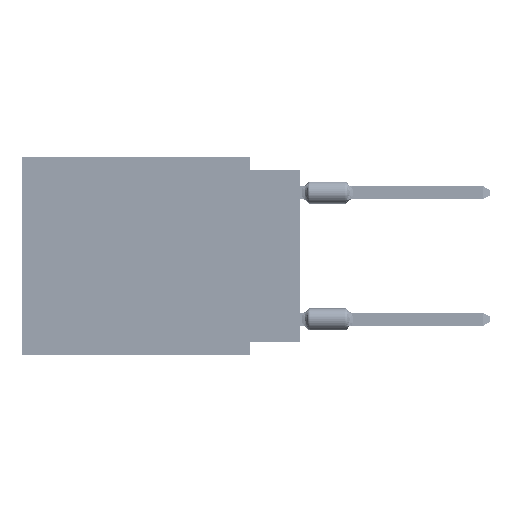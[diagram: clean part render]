
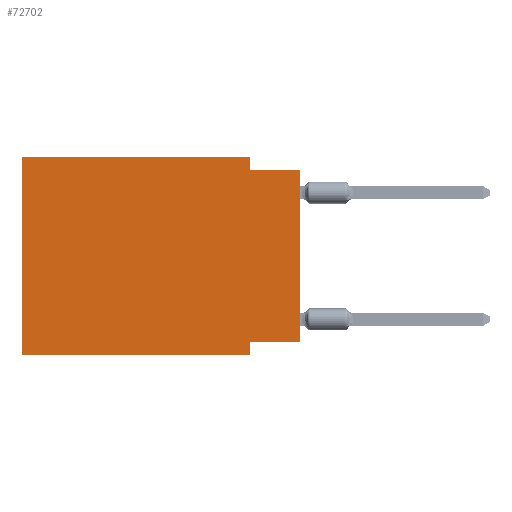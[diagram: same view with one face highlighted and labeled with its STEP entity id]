
A CAD part, left-side view. The second image highlights one B-rep face of the part: STEP entity #72702.
In plain terms, the highlighted planar face has unit normal (-1, 0, 0).
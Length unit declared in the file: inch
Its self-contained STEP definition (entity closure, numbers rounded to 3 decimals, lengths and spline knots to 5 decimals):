
#248 = ORIENTED_EDGE ( 'NONE', *, *, #46616, .F. ) ;
#855 = VERTEX_POINT ( 'NONE', #17338 ) ;
#4907 = EDGE_CURVE ( 'NONE', #21713, #52062, #63877, .T. ) ;
#8021 = VECTOR ( 'NONE', #56955, 39.37008 ) ;
#8079 = VECTOR ( 'NONE', #19343, 39.37008 ) ;
#8705 = DIRECTION ( 'NONE',  ( 0., 0., -1. ) ) ;
#11997 = VERTEX_POINT ( 'NONE', #60979 ) ;
#12090 = VECTOR ( 'NONE', #21885, 39.37008 ) ;
#13390 = ORIENTED_EDGE ( 'NONE', *, *, #50834, .F. ) ;
#13550 = VERTEX_POINT ( 'NONE', #25296 ) ;
#13817 = ORIENTED_EDGE ( 'NONE', *, *, #52555, .T. ) ;
#13846 = CARTESIAN_POINT ( 'NONE',  ( 0., 0., -0.365 ) ) ;
#15242 = AXIS2_PLACEMENT_3D ( 'NONE', #73404, #66898, #30303 ) ;
#16432 = VERTEX_POINT ( 'NONE', #57697 ) ;
#17338 = CARTESIAN_POINT ( 'NONE',  ( 0., 0.1, -0.025 ) ) ;
#18541 = FACE_OUTER_BOUND ( 'NONE', #53073, .T. ) ;
#19343 = DIRECTION ( 'NONE',  ( 0., 0., -1. ) ) ;
#20494 = EDGE_CURVE ( 'NONE', #21713, #43402, #51927, .T. ) ;
#21713 = VERTEX_POINT ( 'NONE', #13846 ) ;
#21885 = DIRECTION ( 'NONE',  ( 0., -1., 0. ) ) ;
#22284 = LINE ( 'NONE', #28752, #12090 ) ;
#22707 = VECTOR ( 'NONE', #46267, 39.37008 ) ;
#23583 = EDGE_CURVE ( 'NONE', #16432, #855, #25038, .T. ) ;
#25038 = LINE ( 'NONE', #44922, #8079 ) ;
#25296 = CARTESIAN_POINT ( 'NONE',  ( 0., 0.55, 0. ) ) ;
#26892 = DIRECTION ( 'NONE',  ( 0., 1., 0. ) ) ;
#27740 = ORIENTED_EDGE ( 'NONE', *, *, #44227, .F. ) ;
#28752 = CARTESIAN_POINT ( 'NONE',  ( 0., 0.55, -0.39 ) ) ;
#28840 = CARTESIAN_POINT ( 'NONE',  ( 0., 0.1, -0.365 ) ) ;
#30303 = DIRECTION ( 'NONE',  ( 0., 0., -1. ) ) ;
#33989 = EDGE_CURVE ( 'NONE', #855, #43402, #34482, .T. ) ;
#34482 = LINE ( 'NONE', #71459, #22707 ) ;
#39446 = LINE ( 'NONE', #63038, #8021 ) ;
#39903 = CARTESIAN_POINT ( 'NONE',  ( 0., 0., -0.365 ) ) ;
#43402 = VERTEX_POINT ( 'NONE', #49380 ) ;
#44103 = VECTOR ( 'NONE', #69834, 39.37008 ) ;
#44227 = EDGE_CURVE ( 'NONE', #11997, #13550, #77237, .T. ) ;
#44922 = CARTESIAN_POINT ( 'NONE',  ( 0., 0.1, 0. ) ) ;
#46267 = DIRECTION ( 'NONE',  ( 0., -1., 0. ) ) ;
#46616 = EDGE_CURVE ( 'NONE', #52062, #60278, #64748, .T. ) ;
#47043 = VECTOR ( 'NONE', #8705, 39.37008 ) ;
#49380 = CARTESIAN_POINT ( 'NONE',  ( 0., 0., -0.025 ) ) ;
#49924 = CARTESIAN_POINT ( 'NONE',  ( 0., 0.1, -0.39 ) ) ;
#50834 = EDGE_CURVE ( 'NONE', #13550, #16432, #39446, .T. ) ;
#51927 = LINE ( 'NONE', #75527, #44103 ) ;
#52062 = VERTEX_POINT ( 'NONE', #28840 ) ;
#52555 = EDGE_CURVE ( 'NONE', #11997, #60278, #22284, .T. ) ;
#52916 = ORIENTED_EDGE ( 'NONE', *, *, #23583, .F. ) ;
#53073 = EDGE_LOOP ( 'NONE', ( #71680, #72666, #52916, #13390, #27740, #13817, #248, #55744 ) ) ;
#55744 = ORIENTED_EDGE ( 'NONE', *, *, #4907, .F. ) ;
#56955 = DIRECTION ( 'NONE',  ( 0., -1., 0. ) ) ;
#57697 = CARTESIAN_POINT ( 'NONE',  ( 0., 0.1, 0. ) ) ;
#59858 = CARTESIAN_POINT ( 'NONE',  ( 0., 0.1, -0.39 ) ) ;
#60278 = VERTEX_POINT ( 'NONE', #49924 ) ;
#60979 = CARTESIAN_POINT ( 'NONE',  ( 0., 0.55, -0.39 ) ) ;
#61595 = PLANE ( 'NONE',  #15242 ) ;
#61635 = VECTOR ( 'NONE', #26892, 39.37008 ) ;
#63038 = CARTESIAN_POINT ( 'NONE',  ( 0., 0.55, 0. ) ) ;
#63877 = LINE ( 'NONE', #39903, #61635 ) ;
#64748 = LINE ( 'NONE', #59858, #47043 ) ;
#66898 = DIRECTION ( 'NONE',  ( 1., 0., 0. ) ) ;
#69834 = DIRECTION ( 'NONE',  ( 0., 0., 1. ) ) ;
#71459 = CARTESIAN_POINT ( 'NONE',  ( 0., 0., -0.025 ) ) ;
#71680 = ORIENTED_EDGE ( 'NONE', *, *, #20494, .T. ) ;
#72666 = ORIENTED_EDGE ( 'NONE', *, *, #33989, .F. ) ;
#72702 = ADVANCED_FACE ( 'NONE', ( #18541 ), #61595, .F. ) ;
#72759 = CARTESIAN_POINT ( 'NONE',  ( 0., 0.55, 0. ) ) ;
#72870 = VECTOR ( 'NONE', #74369, 39.37008 ) ;
#73404 = CARTESIAN_POINT ( 'NONE',  ( 0., 0.55, 0. ) ) ;
#74369 = DIRECTION ( 'NONE',  ( 0., 0., 1. ) ) ;
#75527 = CARTESIAN_POINT ( 'NONE',  ( 0., 0., 0. ) ) ;
#77237 = LINE ( 'NONE', #72759, #72870 ) ;
